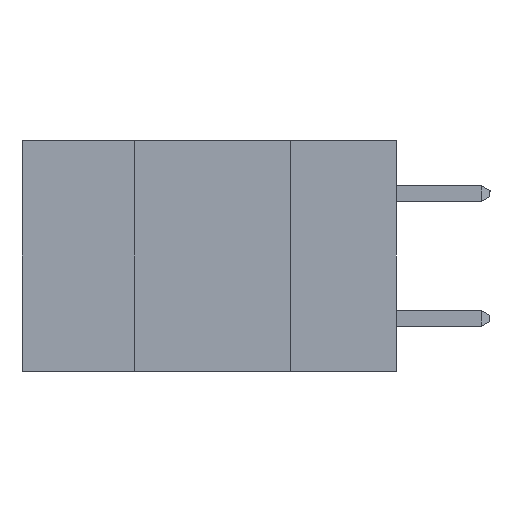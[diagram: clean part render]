
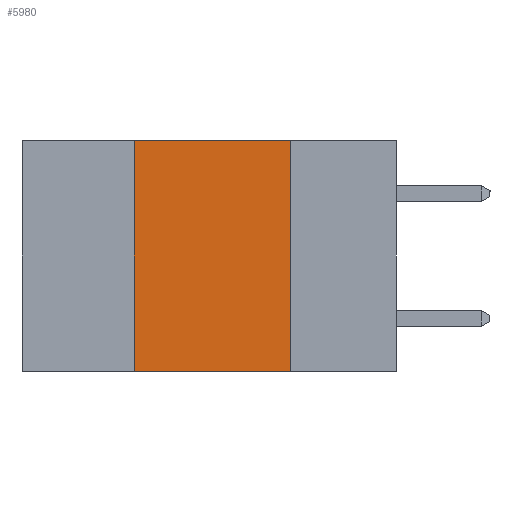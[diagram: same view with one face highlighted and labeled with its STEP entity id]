
A CAD part, left-side view. The second image highlights one B-rep face of the part: STEP entity #5980.
In plain terms, the highlighted planar face has unit normal (-1, 0, 0).
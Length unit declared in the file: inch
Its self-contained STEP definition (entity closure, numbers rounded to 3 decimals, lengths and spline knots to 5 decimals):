
#75 = VECTOR ( 'NONE', #12190, 39.37008 ) ;
#519 = DIRECTION ( 'NONE',  ( 1., 0., 0. ) ) ;
#806 = DIRECTION ( 'NONE',  ( 0., 0., -1. ) ) ;
#891 = FACE_OUTER_BOUND ( 'NONE', #7971, .T. ) ;
#1351 = CARTESIAN_POINT ( 'NONE',  ( 0., 0.17, -0.37 ) ) ;
#1607 = VERTEX_POINT ( 'NONE', #10435 ) ;
#2219 = EDGE_CURVE ( 'NONE', #11746, #1607, #8041, .T. ) ;
#2398 = CARTESIAN_POINT ( 'NONE',  ( 0., 0.6, 0. ) ) ;
#3519 = DIRECTION ( 'NONE',  ( 0., -1., 0. ) ) ;
#3637 = LINE ( 'NONE', #4766, #8407 ) ;
#3716 = DIRECTION ( 'NONE',  ( 0., 0., 1. ) ) ;
#3954 = EDGE_CURVE ( 'NONE', #1607, #11021, #6346, .T. ) ;
#4766 = CARTESIAN_POINT ( 'NONE',  ( 0., 0.17, -0.37 ) ) ;
#5027 = ORIENTED_EDGE ( 'NONE', *, *, #14570, .F. ) ;
#5980 = ADVANCED_FACE ( 'NONE', ( #891 ), #13436, .F. ) ;
#6346 = LINE ( 'NONE', #2398, #9659 ) ;
#7971 = EDGE_LOOP ( 'NONE', ( #5027, #13659, #15254, #17968 ) ) ;
#8041 = LINE ( 'NONE', #11175, #11094 ) ;
#8407 = VECTOR ( 'NONE', #10908, 39.37008 ) ;
#8822 = CARTESIAN_POINT ( 'NONE',  ( 0., 0.17, 0. ) ) ;
#9659 = VECTOR ( 'NONE', #3519, 39.37008 ) ;
#10435 = CARTESIAN_POINT ( 'NONE',  ( 0., 0.42, 0. ) ) ;
#10908 = DIRECTION ( 'NONE',  ( 0., 0., -1. ) ) ;
#11021 = VERTEX_POINT ( 'NONE', #8822 ) ;
#11094 = VECTOR ( 'NONE', #3716, 39.37008 ) ;
#11175 = CARTESIAN_POINT ( 'NONE',  ( 0., 0.42, -0.37 ) ) ;
#11746 = VERTEX_POINT ( 'NONE', #14093 ) ;
#12190 = DIRECTION ( 'NONE',  ( 0., -1., 0. ) ) ;
#13436 = PLANE ( 'NONE',  #16093 ) ;
#13526 = CARTESIAN_POINT ( 'NONE',  ( 0., 0.6, 0. ) ) ;
#13610 = LINE ( 'NONE', #17761, #75 ) ;
#13659 = ORIENTED_EDGE ( 'NONE', *, *, #3954, .F. ) ;
#14093 = CARTESIAN_POINT ( 'NONE',  ( 0., 0.42, -0.37 ) ) ;
#14570 = EDGE_CURVE ( 'NONE', #11021, #15823, #3637, .T. ) ;
#15254 = ORIENTED_EDGE ( 'NONE', *, *, #2219, .F. ) ;
#15823 = VERTEX_POINT ( 'NONE', #1351 ) ;
#16093 = AXIS2_PLACEMENT_3D ( 'NONE', #13526, #519, #806 ) ;
#16917 = EDGE_CURVE ( 'NONE', #11746, #15823, #13610, .T. ) ;
#17761 = CARTESIAN_POINT ( 'NONE',  ( 0., 0.6, -0.37 ) ) ;
#17968 = ORIENTED_EDGE ( 'NONE', *, *, #16917, .T. ) ;
